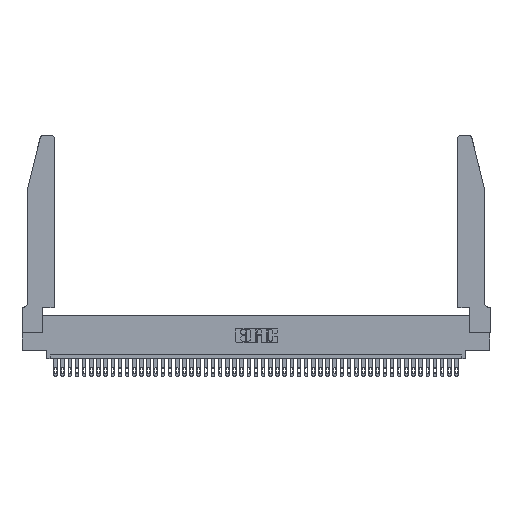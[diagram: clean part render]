
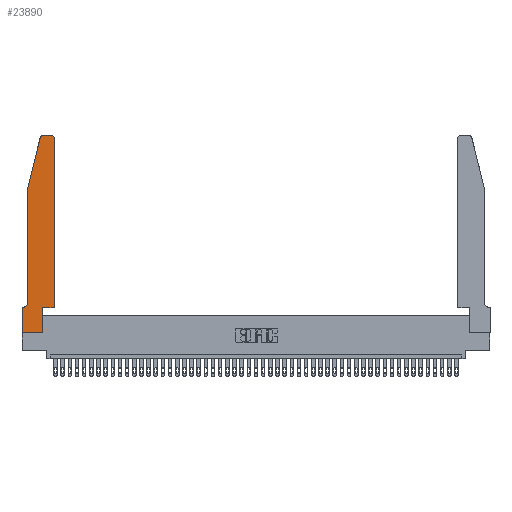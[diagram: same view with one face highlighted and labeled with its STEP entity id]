
A CAD part, top view. The second image highlights one B-rep face of the part: STEP entity #23890.
In plain terms, the highlighted planar face has unit normal (0, 0, 1).
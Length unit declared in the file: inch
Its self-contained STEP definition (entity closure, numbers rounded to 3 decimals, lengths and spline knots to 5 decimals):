
#627 = CARTESIAN_POINT ( 'NONE',  ( 0.284, 2.75, 0.37 ) ) ;
#708 = CARTESIAN_POINT ( 'NONE',  ( 0.0755, 0.42, 0.37 ) ) ;
#1417 = VERTEX_POINT ( 'NONE', #44394 ) ;
#2210 = CARTESIAN_POINT ( 'NONE',  ( 0.2865, 0., 0.37 ) ) ;
#2317 = VERTEX_POINT ( 'NONE', #13079 ) ;
#2573 = DIRECTION ( 'NONE',  ( 0., 1., 0. ) ) ;
#2811 = PLANE ( 'NONE',  #26416 ) ;
#4711 = ORIENTED_EDGE ( 'NONE', *, *, #41461, .T. ) ;
#5066 = CARTESIAN_POINT ( 'NONE',  ( 0., 0., 0.37 ) ) ;
#5154 = VERTEX_POINT ( 'NONE', #18388 ) ;
#5225 = CARTESIAN_POINT ( 'NONE',  ( 0.2865, 0.35, 0.37 ) ) ;
#6053 = CARTESIAN_POINT ( 'NONE',  ( 0.4505, 0.35, 0.37 ) ) ;
#6835 = DIRECTION ( 'NONE',  ( 1., 0., 0. ) ) ;
#7091 = CARTESIAN_POINT ( 'NONE',  ( 0.4205, 2.75, 0.37 ) ) ;
#7254 = VERTEX_POINT ( 'NONE', #5066 ) ;
#7890 = VERTEX_POINT ( 'NONE', #30725 ) ;
#9454 = DIRECTION ( 'NONE',  ( 0., 0., 1. ) ) ;
#9684 = CARTESIAN_POINT ( 'NONE',  ( 0.4505, 0.35, 0.37 ) ) ;
#10453 = VECTOR ( 'NONE', #2573, 39.37008 ) ;
#11072 = ORIENTED_EDGE ( 'NONE', *, *, #17553, .T. ) ;
#11115 = ORIENTED_EDGE ( 'NONE', *, *, #27845, .T. ) ;
#11306 = VERTEX_POINT ( 'NONE', #2210 ) ;
#11325 = CIRCLE ( 'NONE', #21803, 0.07 ) ;
#12140 = DIRECTION ( 'NONE',  ( 1., 0., 0. ) ) ;
#12332 = EDGE_CURVE ( 'NONE', #1417, #7890, #35775, .T. ) ;
#12739 = DIRECTION ( 'NONE',  ( 0., 1., 0. ) ) ;
#12979 = LINE ( 'NONE', #23752, #27259 ) ;
#13079 = CARTESIAN_POINT ( 'NONE',  ( 0.4505, 2.72, 0.37 ) ) ;
#13152 = CARTESIAN_POINT ( 'NONE',  ( 0., 0.35, 0.37 ) ) ;
#13306 = VERTEX_POINT ( 'NONE', #627 ) ;
#14168 = VECTOR ( 'NONE', #30068, 39.37008 ) ;
#14741 = ORIENTED_EDGE ( 'NONE', *, *, #39956, .T. ) ;
#15913 = EDGE_CURVE ( 'NONE', #5154, #32975, #36355, .T. ) ;
#17413 = DIRECTION ( 'NONE',  ( 0., -1., 0. ) ) ;
#17553 = EDGE_CURVE ( 'NONE', #31352, #24267, #43391, .T. ) ;
#18388 = CARTESIAN_POINT ( 'NONE',  ( 0.0055, 0.35, 0.37 ) ) ;
#18613 = VERTEX_POINT ( 'NONE', #708 ) ;
#19610 = ORIENTED_EDGE ( 'NONE', *, *, #25000, .T. ) ;
#19765 = EDGE_CURVE ( 'NONE', #7254, #11306, #24642, .T. ) ;
#19817 = LINE ( 'NONE', #9684, #10453 ) ;
#19905 = EDGE_CURVE ( 'NONE', #24267, #18613, #42320, .T. ) ;
#20169 = ORIENTED_EDGE ( 'NONE', *, *, #15913, .T. ) ;
#20212 = EDGE_CURVE ( 'NONE', #2317, #25875, #29533, .T. ) ;
#20365 = CARTESIAN_POINT ( 'NONE',  ( 0.0755, 2., 0.37 ) ) ;
#21152 = FACE_OUTER_BOUND ( 'NONE', #25669, .T. ) ;
#21241 = EDGE_CURVE ( 'NONE', #11306, #1417, #31179, .T. ) ;
#21695 = CARTESIAN_POINT ( 'NONE',  ( 0.0755, 0.35, 0.37 ) ) ;
#21803 = AXIS2_PLACEMENT_3D ( 'NONE', #39824, #32397, #35959 ) ;
#23405 = CARTESIAN_POINT ( 'NONE',  ( 0., 0., 0.37 ) ) ;
#23605 = DIRECTION ( 'NONE',  ( 1., 0., 0. ) ) ;
#23752 = CARTESIAN_POINT ( 'NONE',  ( 0.2605, 2.75, 0.37 ) ) ;
#23829 = VECTOR ( 'NONE', #17413, 39.37008 ) ;
#23890 = ADVANCED_FACE ( 'NONE', ( #21152 ), #2811, .T. ) ;
#24201 = VECTOR ( 'NONE', #30358, 39.37008 ) ;
#24267 = VERTEX_POINT ( 'NONE', #37005 ) ;
#24466 = DIRECTION ( 'NONE',  ( 0., -1., 0. ) ) ;
#24490 = AXIS2_PLACEMENT_3D ( 'NONE', #26275, #43611, #12140 ) ;
#24642 = LINE ( 'NONE', #23405, #40096 ) ;
#24670 = CARTESIAN_POINT ( 'NONE',  ( 0.4205, 2.72, 0.37 ) ) ;
#25000 = EDGE_CURVE ( 'NONE', #18613, #5154, #11325, .T. ) ;
#25003 = CARTESIAN_POINT ( 'NONE',  ( 0., 0.35, 0.37 ) ) ;
#25669 = EDGE_LOOP ( 'NONE', ( #4711, #11115, #11072, #32120, #19610, #20169, #14741, #27989, #44519, #40133, #34483, #32773 ) ) ;
#25875 = VERTEX_POINT ( 'NONE', #7091 ) ;
#26208 = DIRECTION ( 'NONE',  ( -1., 0., 0. ) ) ;
#26275 = CARTESIAN_POINT ( 'NONE',  ( 0.284, 2.72, 0.37 ) ) ;
#26416 = AXIS2_PLACEMENT_3D ( 'NONE', #13152, #9454, #23605 ) ;
#27259 = VECTOR ( 'NONE', #26208, 39.37008 ) ;
#27334 = DIRECTION ( 'NONE',  ( -1., 0., 0. ) ) ;
#27845 = EDGE_CURVE ( 'NONE', #13306, #31352, #41357, .T. ) ;
#27989 = ORIENTED_EDGE ( 'NONE', *, *, #19765, .T. ) ;
#29142 = CARTESIAN_POINT ( 'NONE',  ( 0.25487, 2.72718, 0.37 ) ) ;
#29533 = CIRCLE ( 'NONE', #36090, 0.03 ) ;
#29911 = CARTESIAN_POINT ( 'NONE',  ( 0.0755, 2., 0.37 ) ) ;
#30068 = DIRECTION ( 'NONE',  ( -0.239, -0.971, 0. ) ) ;
#30358 = DIRECTION ( 'NONE',  ( 1., 0., 0. ) ) ;
#30725 = CARTESIAN_POINT ( 'NONE',  ( 0.4505, 0.35, 0.37 ) ) ;
#30801 = VECTOR ( 'NONE', #27334, 39.37008 ) ;
#31179 = LINE ( 'NONE', #5225, #43353 ) ;
#31352 = VERTEX_POINT ( 'NONE', #29142 ) ;
#31734 = DIRECTION ( 'NONE',  ( 0., 0., 1. ) ) ;
#32120 = ORIENTED_EDGE ( 'NONE', *, *, #19905, .T. ) ;
#32397 = DIRECTION ( 'NONE',  ( 0., 0., -1. ) ) ;
#32773 = ORIENTED_EDGE ( 'NONE', *, *, #20212, .T. ) ;
#32975 = VERTEX_POINT ( 'NONE', #25003 ) ;
#33704 = DIRECTION ( 'NONE',  ( 1., 0., 0. ) ) ;
#34076 = EDGE_CURVE ( 'NONE', #7890, #2317, #19817, .T. ) ;
#34483 = ORIENTED_EDGE ( 'NONE', *, *, #34076, .T. ) ;
#35131 = VECTOR ( 'NONE', #24466, 39.37008 ) ;
#35377 = CARTESIAN_POINT ( 'NONE',  ( 0., 0., 0.37 ) ) ;
#35775 = LINE ( 'NONE', #6053, #24201 ) ;
#35959 = DIRECTION ( 'NONE',  ( -1., 0., 0. ) ) ;
#36090 = AXIS2_PLACEMENT_3D ( 'NONE', #24670, #31734, #6835 ) ;
#36355 = LINE ( 'NONE', #21695, #30801 ) ;
#37005 = CARTESIAN_POINT ( 'NONE',  ( 0.0755, 2., 0.37 ) ) ;
#39824 = CARTESIAN_POINT ( 'NONE',  ( 0.0055, 0.42, 0.37 ) ) ;
#39956 = EDGE_CURVE ( 'NONE', #32975, #7254, #42611, .T. ) ;
#40096 = VECTOR ( 'NONE', #33704, 39.37008 ) ;
#40133 = ORIENTED_EDGE ( 'NONE', *, *, #12332, .T. ) ;
#41357 = CIRCLE ( 'NONE', #24490, 0.03 ) ;
#41461 = EDGE_CURVE ( 'NONE', #25875, #13306, #12979, .T. ) ;
#42320 = LINE ( 'NONE', #20365, #35131 ) ;
#42611 = LINE ( 'NONE', #35377, #23829 ) ;
#43353 = VECTOR ( 'NONE', #12739, 39.37008 ) ;
#43391 = LINE ( 'NONE', #29911, #14168 ) ;
#43611 = DIRECTION ( 'NONE',  ( 0., 0., 1. ) ) ;
#44394 = CARTESIAN_POINT ( 'NONE',  ( 0.2865, 0.35, 0.37 ) ) ;
#44519 = ORIENTED_EDGE ( 'NONE', *, *, #21241, .T. ) ;
